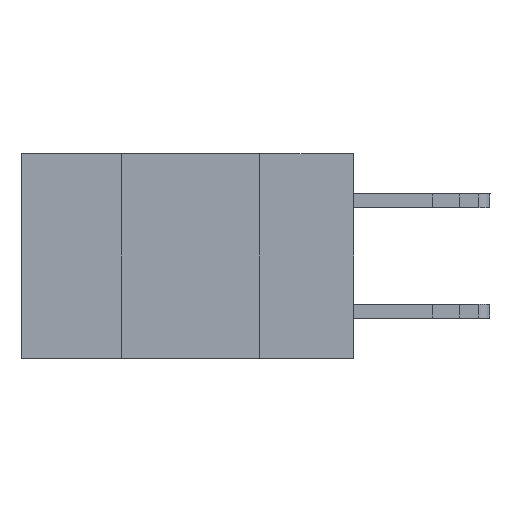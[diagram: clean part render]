
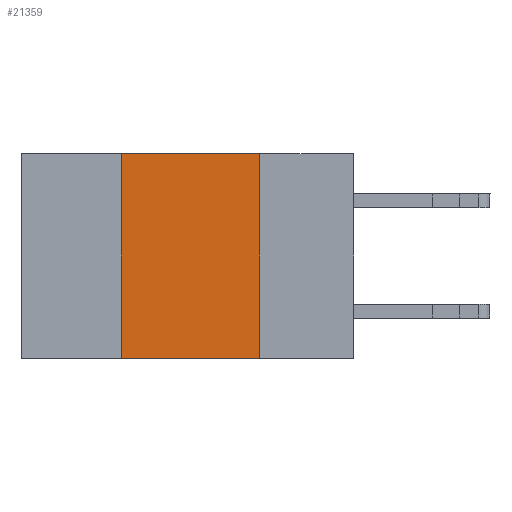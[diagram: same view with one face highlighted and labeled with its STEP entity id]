
A CAD part, left-side view. The second image highlights one B-rep face of the part: STEP entity #21359.
In plain terms, the highlighted planar face has unit normal (-1, 0, 0).
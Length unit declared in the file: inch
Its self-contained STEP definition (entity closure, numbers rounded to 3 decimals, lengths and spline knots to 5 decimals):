
#76 = DIRECTION ( 'NONE',  ( 0., 0., -1. ) ) ;
#222 = CARTESIAN_POINT ( 'NONE',  ( 0., 0.6, -0.37 ) ) ;
#678 = CARTESIAN_POINT ( 'NONE',  ( 0., 0.42, 0. ) ) ;
#790 = EDGE_CURVE ( 'NONE', #18276, #19401, #18454, .T. ) ;
#1638 = VERTEX_POINT ( 'NONE', #24326 ) ;
#2248 = VECTOR ( 'NONE', #12225, 39.37008 ) ;
#3065 = VECTOR ( 'NONE', #12497, 39.37008 ) ;
#4384 = ORIENTED_EDGE ( 'NONE', *, *, #790, .F. ) ;
#5865 = CARTESIAN_POINT ( 'NONE',  ( 0., 0.6, 0. ) ) ;
#6198 = EDGE_CURVE ( 'NONE', #1638, #9220, #6395, .T. ) ;
#6240 = LINE ( 'NONE', #23343, #2248 ) ;
#6395 = LINE ( 'NONE', #18313, #20413 ) ;
#7144 = CARTESIAN_POINT ( 'NONE',  ( 0., 0.42, -0.37 ) ) ;
#7396 = ORIENTED_EDGE ( 'NONE', *, *, #19322, .F. ) ;
#7427 = ORIENTED_EDGE ( 'NONE', *, *, #18574, .T. ) ;
#8599 = FACE_OUTER_BOUND ( 'NONE', #21916, .T. ) ;
#9220 = VERTEX_POINT ( 'NONE', #13453 ) ;
#10815 = DIRECTION ( 'NONE',  ( 0., 0., -1. ) ) ;
#11803 = DIRECTION ( 'NONE',  ( 1., 0., 0. ) ) ;
#12225 = DIRECTION ( 'NONE',  ( 0., -1., 0. ) ) ;
#12497 = DIRECTION ( 'NONE',  ( 0., 0., 1. ) ) ;
#13040 = AXIS2_PLACEMENT_3D ( 'NONE', #5865, #11803, #76 ) ;
#13453 = CARTESIAN_POINT ( 'NONE',  ( 0., 0.17, -0.37 ) ) ;
#13875 = DIRECTION ( 'NONE',  ( 0., -1., 0. ) ) ;
#14704 = ORIENTED_EDGE ( 'NONE', *, *, #6198, .F. ) ;
#14953 = CARTESIAN_POINT ( 'NONE',  ( 0., 0.42, 0. ) ) ;
#18276 = VERTEX_POINT ( 'NONE', #7144 ) ;
#18313 = CARTESIAN_POINT ( 'NONE',  ( 0., 0.17, 0. ) ) ;
#18454 = LINE ( 'NONE', #14953, #3065 ) ;
#18574 = EDGE_CURVE ( 'NONE', #18276, #9220, #23417, .T. ) ;
#18592 = VECTOR ( 'NONE', #13875, 39.37008 ) ;
#19277 = PLANE ( 'NONE',  #13040 ) ;
#19322 = EDGE_CURVE ( 'NONE', #19401, #1638, #6240, .T. ) ;
#19401 = VERTEX_POINT ( 'NONE', #678 ) ;
#20413 = VECTOR ( 'NONE', #10815, 39.37008 ) ;
#21359 = ADVANCED_FACE ( 'NONE', ( #8599 ), #19277, .F. ) ;
#21916 = EDGE_LOOP ( 'NONE', ( #14704, #7396, #4384, #7427 ) ) ;
#23343 = CARTESIAN_POINT ( 'NONE',  ( 0., 0.6, 0. ) ) ;
#23417 = LINE ( 'NONE', #222, #18592 ) ;
#24326 = CARTESIAN_POINT ( 'NONE',  ( 0., 0.17, 0. ) ) ;
